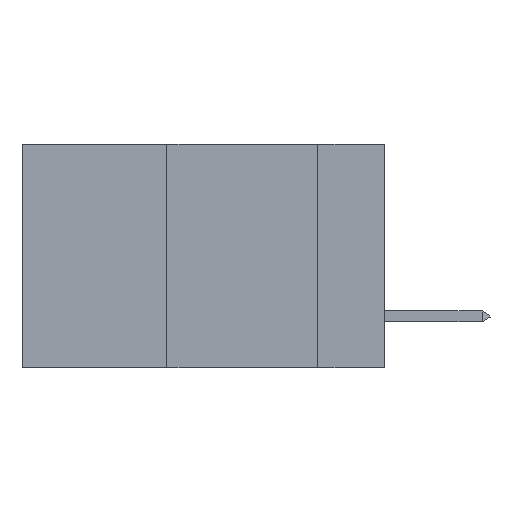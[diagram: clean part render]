
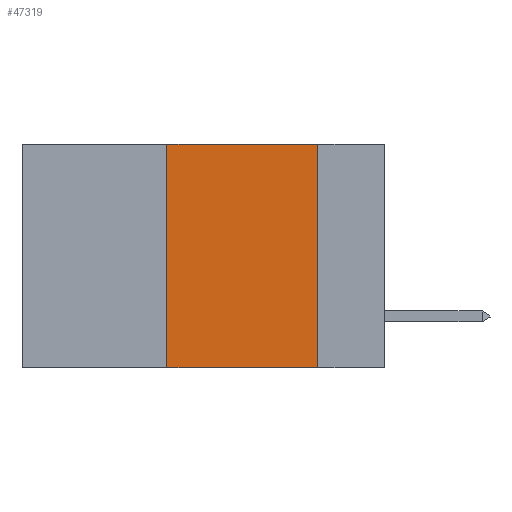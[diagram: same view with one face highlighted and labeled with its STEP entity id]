
A CAD part, left-side view. The second image highlights one B-rep face of the part: STEP entity #47319.
In plain terms, the highlighted planar face has unit normal (-1, 0, 0).
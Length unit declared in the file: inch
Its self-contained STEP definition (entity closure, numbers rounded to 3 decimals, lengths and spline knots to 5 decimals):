
#2983 = CARTESIAN_POINT ( 'NONE',  ( 0., 0.11, 0. ) ) ;
#7510 = LINE ( 'NONE', #44241, #30642 ) ;
#9058 = EDGE_CURVE ( 'NONE', #50234, #19467, #29281, .T. ) ;
#11385 = EDGE_CURVE ( 'NONE', #50395, #45013, #24799, .T. ) ;
#12790 = CARTESIAN_POINT ( 'NONE',  ( 0., 0.6, 0. ) ) ;
#13026 = CARTESIAN_POINT ( 'NONE',  ( 0., 0.6, -0.37 ) ) ;
#13560 = EDGE_CURVE ( 'NONE', #45013, #50234, #7510, .T. ) ;
#16998 = CARTESIAN_POINT ( 'NONE',  ( 0., 0.11, -0.37 ) ) ;
#18114 = DIRECTION ( 'NONE',  ( 0., 0., -1. ) ) ;
#19467 = VERTEX_POINT ( 'NONE', #16998 ) ;
#22346 = VECTOR ( 'NONE', #23421, 39.37008 ) ;
#23051 = LINE ( 'NONE', #13026, #50482 ) ;
#23421 = DIRECTION ( 'NONE',  ( 0., 0., 1. ) ) ;
#23964 = PLANE ( 'NONE',  #32764 ) ;
#24799 = LINE ( 'NONE', #46788, #22346 ) ;
#24876 = ORIENTED_EDGE ( 'NONE', *, *, #11385, .F. ) ;
#28219 = DIRECTION ( 'NONE',  ( 0., -1., 0. ) ) ;
#28574 = DIRECTION ( 'NONE',  ( 1., 0., 0. ) ) ;
#29281 = LINE ( 'NONE', #2983, #33552 ) ;
#30642 = VECTOR ( 'NONE', #28219, 39.37008 ) ;
#31250 = CARTESIAN_POINT ( 'NONE',  ( 0., 0.36, -0.37 ) ) ;
#32047 = EDGE_LOOP ( 'NONE', ( #41966, #37850, #24876, #40813 ) ) ;
#32581 = DIRECTION ( 'NONE',  ( 0., -1., 0. ) ) ;
#32764 = AXIS2_PLACEMENT_3D ( 'NONE', #12790, #28574, #36255 ) ;
#33552 = VECTOR ( 'NONE', #18114, 39.37008 ) ;
#35594 = EDGE_CURVE ( 'NONE', #50395, #19467, #23051, .T. ) ;
#36255 = DIRECTION ( 'NONE',  ( 0., 0., -1. ) ) ;
#37850 = ORIENTED_EDGE ( 'NONE', *, *, #13560, .F. ) ;
#39120 = FACE_OUTER_BOUND ( 'NONE', #32047, .T. ) ;
#40813 = ORIENTED_EDGE ( 'NONE', *, *, #35594, .T. ) ;
#41966 = ORIENTED_EDGE ( 'NONE', *, *, #9058, .F. ) ;
#44241 = CARTESIAN_POINT ( 'NONE',  ( 0., 0.6, 0. ) ) ;
#45013 = VERTEX_POINT ( 'NONE', #45241 ) ;
#45241 = CARTESIAN_POINT ( 'NONE',  ( 0., 0.36, 0. ) ) ;
#46788 = CARTESIAN_POINT ( 'NONE',  ( 0., 0.36, 0. ) ) ;
#47319 = ADVANCED_FACE ( 'NONE', ( #39120 ), #23964, .F. ) ;
#48478 = CARTESIAN_POINT ( 'NONE',  ( 0., 0.11, 0. ) ) ;
#50234 = VERTEX_POINT ( 'NONE', #48478 ) ;
#50395 = VERTEX_POINT ( 'NONE', #31250 ) ;
#50482 = VECTOR ( 'NONE', #32581, 39.37008 ) ;
